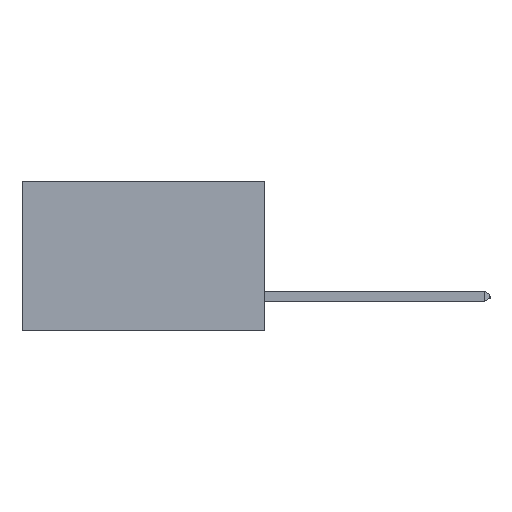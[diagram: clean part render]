
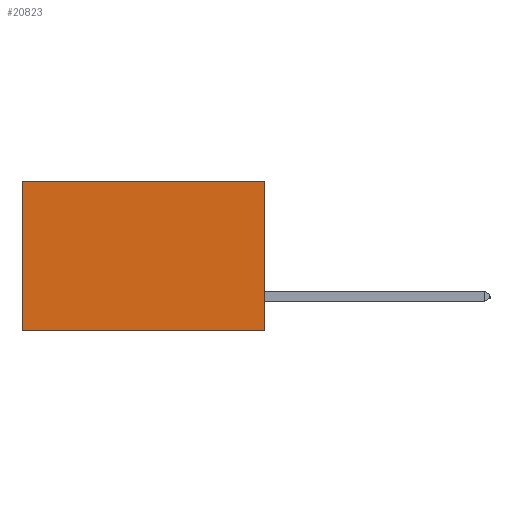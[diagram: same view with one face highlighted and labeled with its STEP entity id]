
A CAD part, left-side view. The second image highlights one B-rep face of the part: STEP entity #20823.
In plain terms, the highlighted planar face has unit normal (-1, 0, 0).
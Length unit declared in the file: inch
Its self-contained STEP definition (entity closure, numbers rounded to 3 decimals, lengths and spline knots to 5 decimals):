
#220 = CARTESIAN_POINT ( 'NONE',  ( 0.298, 0.6, -0.37 ) ) ;
#428 = VECTOR ( 'NONE', #22684, 39.37008 ) ;
#473 = VECTOR ( 'NONE', #13412, 39.37008 ) ;
#579 = DIRECTION ( 'NONE',  ( 1., 0., 0. ) ) ;
#990 = ORIENTED_EDGE ( 'NONE', *, *, #10090, .F. ) ;
#1140 = LINE ( 'NONE', #25680, #473 ) ;
#2570 = CARTESIAN_POINT ( 'NONE',  ( 0.298, 0., 0. ) ) ;
#3438 = VERTEX_POINT ( 'NONE', #20180 ) ;
#4379 = LINE ( 'NONE', #5288, #19558 ) ;
#5288 = CARTESIAN_POINT ( 'NONE',  ( 0.298, 0., 0. ) ) ;
#7230 = CARTESIAN_POINT ( 'NONE',  ( 0.298, 0., 0. ) ) ;
#9271 = DIRECTION ( 'NONE',  ( 0., 1., 0. ) ) ;
#9732 = LINE ( 'NONE', #7230, #25484 ) ;
#9777 = CARTESIAN_POINT ( 'NONE',  ( 0.298, 0.6, 0. ) ) ;
#9829 = VERTEX_POINT ( 'NONE', #9777 ) ;
#10090 = EDGE_CURVE ( 'NONE', #20528, #3438, #4379, .T. ) ;
#11995 = CARTESIAN_POINT ( 'NONE',  ( 0.298, 0., 0. ) ) ;
#13267 = FACE_OUTER_BOUND ( 'NONE', #25768, .T. ) ;
#13412 = DIRECTION ( 'NONE',  ( 0., 1., 0. ) ) ;
#13709 = ORIENTED_EDGE ( 'NONE', *, *, #17903, .F. ) ;
#14014 = VERTEX_POINT ( 'NONE', #220 ) ;
#15070 = DIRECTION ( 'NONE',  ( 0., 0., -1. ) ) ;
#17903 = EDGE_CURVE ( 'NONE', #3438, #14014, #1140, .T. ) ;
#18787 = EDGE_CURVE ( 'NONE', #9829, #14014, #21147, .T. ) ;
#19558 = VECTOR ( 'NONE', #21812, 39.37008 ) ;
#20180 = CARTESIAN_POINT ( 'NONE',  ( 0.298, 0., -0.37 ) ) ;
#20296 = EDGE_CURVE ( 'NONE', #20528, #9829, #9732, .T. ) ;
#20528 = VERTEX_POINT ( 'NONE', #11995 ) ;
#20579 = CARTESIAN_POINT ( 'NONE',  ( 0.298, 0.6, 0. ) ) ;
#20823 = ADVANCED_FACE ( 'NONE', ( #13267 ), #23267, .F. ) ;
#20915 = ORIENTED_EDGE ( 'NONE', *, *, #20296, .T. ) ;
#21147 = LINE ( 'NONE', #20579, #428 ) ;
#21742 = ORIENTED_EDGE ( 'NONE', *, *, #18787, .T. ) ;
#21812 = DIRECTION ( 'NONE',  ( 0., 0., -1. ) ) ;
#22684 = DIRECTION ( 'NONE',  ( 0., 0., -1. ) ) ;
#23267 = PLANE ( 'NONE',  #25990 ) ;
#25484 = VECTOR ( 'NONE', #9271, 39.37008 ) ;
#25680 = CARTESIAN_POINT ( 'NONE',  ( 0.298, 0., -0.37 ) ) ;
#25768 = EDGE_LOOP ( 'NONE', ( #21742, #13709, #990, #20915 ) ) ;
#25990 = AXIS2_PLACEMENT_3D ( 'NONE', #2570, #579, #15070 ) ;
